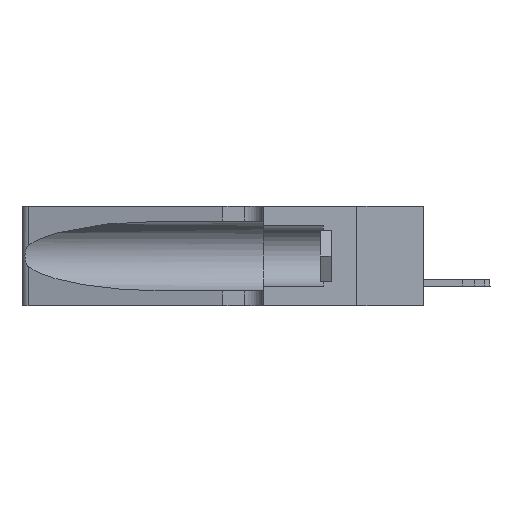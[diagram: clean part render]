
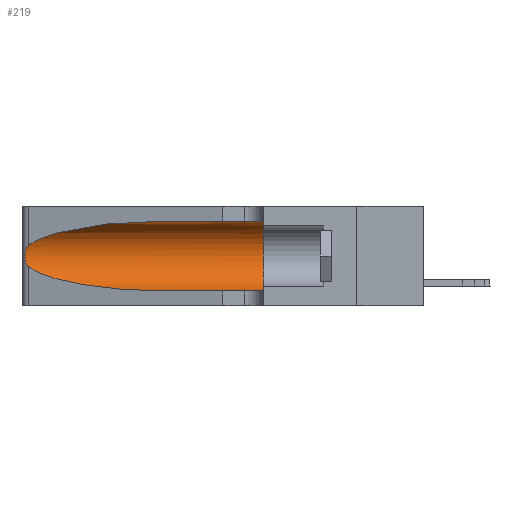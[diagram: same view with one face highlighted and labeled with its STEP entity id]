
A CAD part, left-side view. The second image highlights one B-rep face of the part: STEP entity #219.
In plain terms, the highlighted cylindrical face has radius 3.308 mm (diameter 6.617 mm), a partial arc.
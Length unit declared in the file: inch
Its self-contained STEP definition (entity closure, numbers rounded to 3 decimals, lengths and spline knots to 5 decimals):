
#30 = CARTESIAN_POINT ( 'NONE',  ( 0.25854, 1.2359, 0.20912 ) ) ;
#219 = ADVANCED_FACE ( 'NONE', ( #12216 ), #7429, .F. ) ;
#562 = EDGE_CURVE ( 'NONE', #15530, #7684, #9596, .T. ) ;
#690 = B_SPLINE_CURVE_WITH_KNOTS ( 'NONE', 3,
 ( #14916, #3055, #13138, #11264, #30, #21872, #13837, #3628, #8859, #15537, #2092, #15682, #18384, #21697 ),
 .UNSPECIFIED., .F., .F.,
 ( 4, 2, 2, 2, 2, 2, 4 ),
 ( 0., 0.00027, 0.00053, 0.00107, 0.0016, 0.00187, 0.00214 ),
 .UNSPECIFIED. ) ;
#826 = ORIENTED_EDGE ( 'NONE', *, *, #15699, .F. ) ;
#1015 = EDGE_CURVE ( 'NONE', #4315, #7684, #6098, .T. ) ;
#1428 = ORIENTED_EDGE ( 'NONE', *, *, #19314, .T. ) ;
#1977 = CARTESIAN_POINT ( 'NONE',  ( 0.1305, 1.61858, 0.05475 ) ) ;
#2092 = CARTESIAN_POINT ( 'NONE',  ( 0.25789, 1.23486, 0.15765 ) ) ;
#2428 = EDGE_CURVE ( 'NONE', #17838, #7015, #690, .T. ) ;
#3055 = CARTESIAN_POINT ( 'NONE',  ( 0.25555, 1.22994, 0.2215 ) ) ;
#3364 = CARTESIAN_POINT ( 'NONE',  ( 0.1305, 0.35, 0.31525 ) ) ;
#3628 = CARTESIAN_POINT ( 'NONE',  ( 0.26075, 1.23896, 0.178 ) ) ;
#3844 = ORIENTED_EDGE ( 'NONE', *, *, #2428, .T. ) ;
#4256 = AXIS2_PLACEMENT_3D ( 'NONE', #17809, #7658, #4526 ) ;
#4315 = VERTEX_POINT ( 'NONE', #3364 ) ;
#4526 = DIRECTION ( 'NONE',  ( 0., 0., -1. ) ) ;
#5119 = CARTESIAN_POINT ( 'NONE',  ( 0.1305, 0.72297, 0.31525 ) ) ;
#5942 = VECTOR ( 'NONE', #18536, 39.37008 ) ;
#6050 = VERTEX_POINT ( 'NONE', #15677 ) ;
#6098 = CIRCLE ( 'NONE', #12989, 0.13025 ) ;
#7015 = VERTEX_POINT ( 'NONE', #12647 ) ;
#7181 = ORIENTED_EDGE ( 'NONE', *, *, #21674, .T. ) ;
#7282 =( BOUNDED_CURVE ( )  B_SPLINE_CURVE ( 3, ( #5119, #18741, #20524, #15292 ),
 .UNSPECIFIED., .F., .T. ) 
 B_SPLINE_CURVE_WITH_KNOTS ( ( 4, 4 ),
 ( 1.5708, 2.84003 ),
 .UNSPECIFIED. ) 
 CURVE ( )  GEOMETRIC_REPRESENTATION_ITEM ( )  RATIONAL_B_SPLINE_CURVE ( ( 1., 0.87, 0.87, 1. ) ) 
 REPRESENTATION_ITEM ( '' )  );
#7429 = CYLINDRICAL_SURFACE ( 'NONE', #4256, 0.13025 ) ;
#7658 = DIRECTION ( 'NONE',  ( 0., -1., 0. ) ) ;
#7684 = VERTEX_POINT ( 'NONE', #16298 ) ;
#8062 = DIRECTION ( 'NONE',  ( 0., 1., 0. ) ) ;
#8765 = EDGE_LOOP ( 'NONE', ( #1428, #3844, #7181, #10912, #9619, #826 ) ) ;
#8859 = CARTESIAN_POINT ( 'NONE',  ( 0.26017, 1.23833, 0.17102 ) ) ;
#9140 = LINE ( 'NONE', #13445, #5942 ) ;
#9302 = CARTESIAN_POINT ( 'NONE',  ( 0.18966, 0.96281, 0.05475 ) ) ;
#9596 = LINE ( 'NONE', #1977, #17013 ) ;
#9619 = ORIENTED_EDGE ( 'NONE', *, *, #1015, .F. ) ;
#10064 = CARTESIAN_POINT ( 'NONE',  ( 0.25487, 1.22718, 0.22369 ) ) ;
#10708 = CARTESIAN_POINT ( 'NONE',  ( 0.25487, 1.22718, 0.14631 ) ) ;
#10912 = ORIENTED_EDGE ( 'NONE', *, *, #562, .T. ) ;
#10986 = CARTESIAN_POINT ( 'NONE',  ( 0.1305, 0.72297, 0.05475 ) ) ;
#11264 = CARTESIAN_POINT ( 'NONE',  ( 0.25787, 1.23484, 0.2124 ) ) ;
#12216 = FACE_OUTER_BOUND ( 'NONE', #8765, .T. ) ;
#12647 = CARTESIAN_POINT ( 'NONE',  ( 0.25487, 1.22718, 0.14631 ) ) ;
#12989 = AXIS2_PLACEMENT_3D ( 'NONE', #21366, #8062, #16484 ) ;
#13138 = CARTESIAN_POINT ( 'NONE',  ( 0.25639, 1.23184, 0.21858 ) ) ;
#13445 = CARTESIAN_POINT ( 'NONE',  ( 0.1305, 1.61858, 0.31525 ) ) ;
#13837 = CARTESIAN_POINT ( 'NONE',  ( 0.26075, 1.23896, 0.19203 ) ) ;
#13874 = DIRECTION ( 'NONE',  ( 0., -1., 0. ) ) ;
#14916 = CARTESIAN_POINT ( 'NONE',  ( 0.25487, 1.22718, 0.22369 ) ) ;
#15186 =( BOUNDED_CURVE ( )  B_SPLINE_CURVE ( 3, ( #10708, #15822, #9302, #21248 ),
 .UNSPECIFIED., .F., .F. ) 
 B_SPLINE_CURVE_WITH_KNOTS ( ( 4, 4 ),
 ( 3.44316, 4.71239 ),
 .UNSPECIFIED. ) 
 CURVE ( )  GEOMETRIC_REPRESENTATION_ITEM ( )  RATIONAL_B_SPLINE_CURVE ( ( 1., 0.87, 0.87, 1. ) ) 
 REPRESENTATION_ITEM ( '' )  );
#15292 = CARTESIAN_POINT ( 'NONE',  ( 0.25487, 1.22718, 0.22369 ) ) ;
#15530 = VERTEX_POINT ( 'NONE', #10986 ) ;
#15537 = CARTESIAN_POINT ( 'NONE',  ( 0.25856, 1.23593, 0.16098 ) ) ;
#15677 = CARTESIAN_POINT ( 'NONE',  ( 0.1305, 0.72297, 0.31525 ) ) ;
#15682 = CARTESIAN_POINT ( 'NONE',  ( 0.25639, 1.23186, 0.15144 ) ) ;
#15699 = EDGE_CURVE ( 'NONE', #6050, #4315, #9140, .T. ) ;
#15822 = CARTESIAN_POINT ( 'NONE',  ( 0.2373, 1.15595, 0.08982 ) ) ;
#16298 = CARTESIAN_POINT ( 'NONE',  ( 0.1305, 0.35, 0.05475 ) ) ;
#16484 = DIRECTION ( 'NONE',  ( 0., 0., 1. ) ) ;
#17013 = VECTOR ( 'NONE', #13874, 39.37008 ) ;
#17809 = CARTESIAN_POINT ( 'NONE',  ( 0.1305, 1.61858, 0.185 ) ) ;
#17838 = VERTEX_POINT ( 'NONE', #10064 ) ;
#18384 = CARTESIAN_POINT ( 'NONE',  ( 0.25555, 1.22993, 0.14849 ) ) ;
#18536 = DIRECTION ( 'NONE',  ( 0., -1., 0. ) ) ;
#18741 = CARTESIAN_POINT ( 'NONE',  ( 0.18966, 0.96281, 0.31525 ) ) ;
#19314 = EDGE_CURVE ( 'NONE', #6050, #17838, #7282, .T. ) ;
#20524 = CARTESIAN_POINT ( 'NONE',  ( 0.2373, 1.15595, 0.28018 ) ) ;
#21248 = CARTESIAN_POINT ( 'NONE',  ( 0.1305, 0.72297, 0.05475 ) ) ;
#21366 = CARTESIAN_POINT ( 'NONE',  ( 0.1305, 0.35, 0.185 ) ) ;
#21674 = EDGE_CURVE ( 'NONE', #7015, #15530, #15186, .T. ) ;
#21697 = CARTESIAN_POINT ( 'NONE',  ( 0.25487, 1.22718, 0.14631 ) ) ;
#21872 = CARTESIAN_POINT ( 'NONE',  ( 0.26018, 1.23835, 0.19895 ) ) ;
